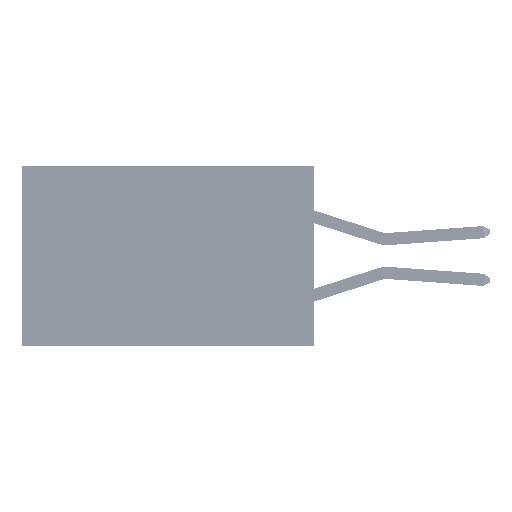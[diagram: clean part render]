
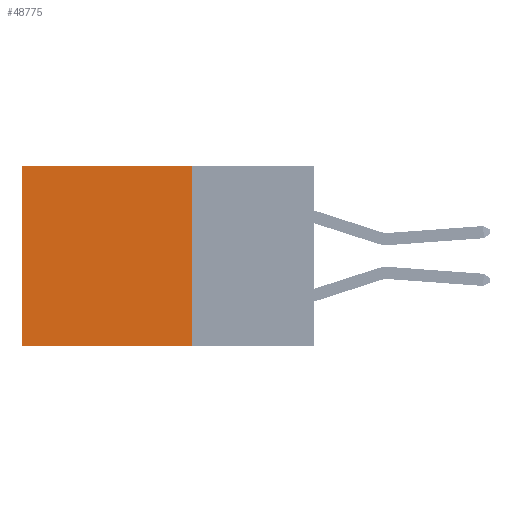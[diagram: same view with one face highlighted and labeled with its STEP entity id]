
A CAD part, left-side view. The second image highlights one B-rep face of the part: STEP entity #48775.
In plain terms, the highlighted planar face has unit normal (-1, 0, 0).
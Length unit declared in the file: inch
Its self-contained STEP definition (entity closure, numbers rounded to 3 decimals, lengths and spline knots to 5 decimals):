
#783 = ORIENTED_EDGE ( 'NONE', *, *, #16204, .T. ) ;
#3034 = VECTOR ( 'NONE', #39670, 39.37008 ) ;
#3874 = DIRECTION ( 'NONE',  ( 1., 0., 0. ) ) ;
#4066 = EDGE_CURVE ( 'NONE', #12940, #4590, #13429, .T. ) ;
#4590 = VERTEX_POINT ( 'NONE', #50466 ) ;
#4649 = CARTESIAN_POINT ( 'NONE',  ( 0.2875, 0.6, 0. ) ) ;
#4772 = LINE ( 'NONE', #13330, #15831 ) ;
#6427 = FACE_OUTER_BOUND ( 'NONE', #9342, .T. ) ;
#6853 = CARTESIAN_POINT ( 'NONE',  ( 0.2875, 0.25, -0.37 ) ) ;
#8145 = PLANE ( 'NONE',  #29704 ) ;
#9342 = EDGE_LOOP ( 'NONE', ( #14314, #22145, #27522, #783 ) ) ;
#9513 = CARTESIAN_POINT ( 'NONE',  ( 0.2875, 0.25, 0. ) ) ;
#9543 = LINE ( 'NONE', #9513, #28444 ) ;
#12068 = VERTEX_POINT ( 'NONE', #26155 ) ;
#12070 = VERTEX_POINT ( 'NONE', #6853 ) ;
#12940 = VERTEX_POINT ( 'NONE', #4649 ) ;
#13330 = CARTESIAN_POINT ( 'NONE',  ( 0.2875, 0.25, 0. ) ) ;
#13429 = LINE ( 'NONE', #39333, #3034 ) ;
#14314 = ORIENTED_EDGE ( 'NONE', *, *, #4066, .T. ) ;
#15831 = VECTOR ( 'NONE', #40148, 39.37008 ) ;
#16204 = EDGE_CURVE ( 'NONE', #12068, #12940, #9543, .T. ) ;
#16874 = EDGE_CURVE ( 'NONE', #12070, #4590, #40317, .T. ) ;
#17562 = EDGE_CURVE ( 'NONE', #12068, #12070, #4772, .T. ) ;
#19921 = DIRECTION ( 'NONE',  ( 0., 0., -1. ) ) ;
#21639 = DIRECTION ( 'NONE',  ( 0., 1., 0. ) ) ;
#22145 = ORIENTED_EDGE ( 'NONE', *, *, #16874, .F. ) ;
#26155 = CARTESIAN_POINT ( 'NONE',  ( 0.2875, 0.25, 0. ) ) ;
#27522 = ORIENTED_EDGE ( 'NONE', *, *, #17562, .F. ) ;
#28444 = VECTOR ( 'NONE', #21639, 39.37008 ) ;
#29704 = AXIS2_PLACEMENT_3D ( 'NONE', #34783, #3874, #19921 ) ;
#33328 = DIRECTION ( 'NONE',  ( 0., 1., 0. ) ) ;
#34783 = CARTESIAN_POINT ( 'NONE',  ( 0.2875, 0.25, 0. ) ) ;
#39333 = CARTESIAN_POINT ( 'NONE',  ( 0.2875, 0.6, 0. ) ) ;
#39670 = DIRECTION ( 'NONE',  ( 0., 0., -1. ) ) ;
#40038 = CARTESIAN_POINT ( 'NONE',  ( 0.2875, 0.25, -0.37 ) ) ;
#40148 = DIRECTION ( 'NONE',  ( 0., 0., -1. ) ) ;
#40317 = LINE ( 'NONE', #40038, #45786 ) ;
#45786 = VECTOR ( 'NONE', #33328, 39.37008 ) ;
#48775 = ADVANCED_FACE ( 'NONE', ( #6427 ), #8145, .F. ) ;
#50466 = CARTESIAN_POINT ( 'NONE',  ( 0.2875, 0.6, -0.37 ) ) ;
